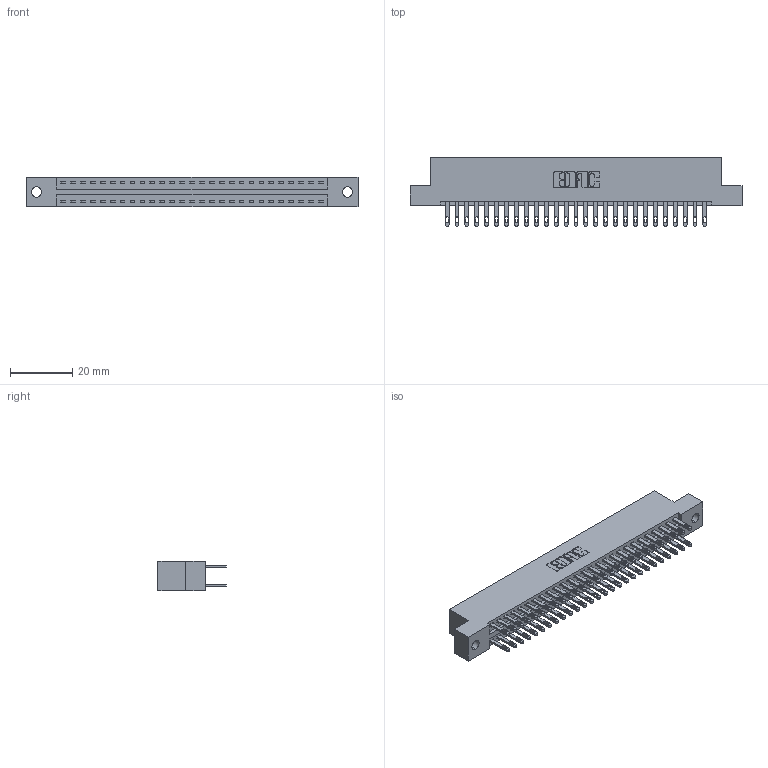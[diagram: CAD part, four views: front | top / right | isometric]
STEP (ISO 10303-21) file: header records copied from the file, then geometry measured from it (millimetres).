
FILE_DESCRIPTION (( 'STEP AP203' ), '1' );
FILE_NAME ('346-054-500-202.STEP', '2018-08-28T00:41:46', ( '' ), ( '' ), 'SwSTEP 2.0', 'SolidWorks 2016', '' );
FILE_SCHEMA (( 'CONFIG_CONTROL_DESIGN' ));
Length unit declared in the file: inch
Products named in the file (3): 346 Part_Flush Mounting Lugs - 0.128 Dia; 345-292-001_345-293-100; 346-054-500-202
Assembly tree (55 placements, depth 2):
  346-054-500-202
    346 Part_Flush Mounting Lugs - 0.128 Dia
    345-292-001_345-293-100  x54
Bounding box: 106.3 x 21.84 x 9.4 mm (x, y, z)
Volume: 10377.3 mm3; surface area: 14324.5 mm2
Topology: 55 solids, 55 shells, 2714 faces, 8267 edges, 5510 vertices
Faces by surface type: plane 1642, cylinder 1072
Entity records: 19573 total; most frequent: CARTESIAN_POINT 3244, ORIENTED_EDGE 3178, DIRECTION 2913, EDGE_CURVE 1589, LINE 1345, VECTOR 1345, VERTEX_POINT 1058, AXIS2_PLACEMENT_3D 784
